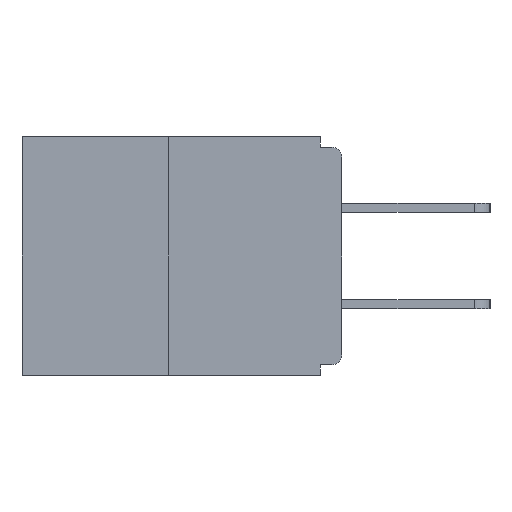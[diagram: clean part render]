
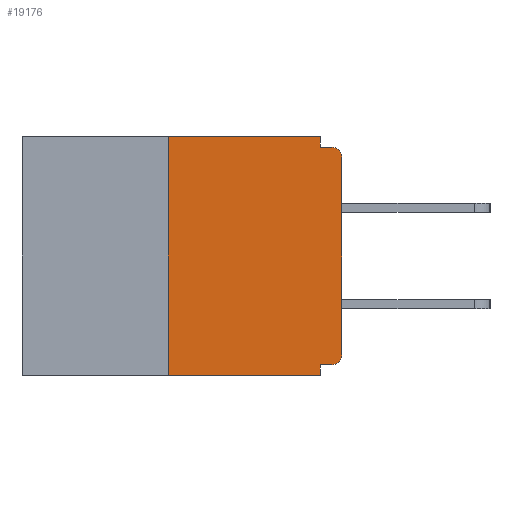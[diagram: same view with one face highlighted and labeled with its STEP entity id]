
A CAD part, left-side view. The second image highlights one B-rep face of the part: STEP entity #19176.
In plain terms, the highlighted planar face has unit normal (-1, 0, 0).
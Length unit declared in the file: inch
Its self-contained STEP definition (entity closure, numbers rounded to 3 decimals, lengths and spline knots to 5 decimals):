
#109 = VECTOR ( 'NONE', #12124, 39.37008 ) ;
#890 = DIRECTION ( 'NONE',  ( 0., 0., -1. ) ) ;
#1224 = VERTEX_POINT ( 'NONE', #20344 ) ;
#1294 = DIRECTION ( 'NONE',  ( 0., -1., 0. ) ) ;
#1757 = ORIENTED_EDGE ( 'NONE', *, *, #17096, .F. ) ;
#1772 = VERTEX_POINT ( 'NONE', #9847 ) ;
#1871 = CARTESIAN_POINT ( 'NONE',  ( 0., 0.46, -0.343 ) ) ;
#2047 = EDGE_CURVE ( 'NONE', #1772, #11818, #23178, .T. ) ;
#2252 = VERTEX_POINT ( 'NONE', #16601 ) ;
#2496 = CARTESIAN_POINT ( 'NONE',  ( 0., 0.015, -0.313 ) ) ;
#2564 = LINE ( 'NONE', #8183, #4224 ) ;
#2820 = EDGE_LOOP ( 'NONE', ( #18465, #4068, #4355, #13558, #8547, #20188, #20332, #4637, #1757, #14184 ) ) ;
#2982 = CARTESIAN_POINT ( 'NONE',  ( 0., 0.015, -0.015 ) ) ;
#3089 = CARTESIAN_POINT ( 'NONE',  ( 0., 0.46, 0. ) ) ;
#3506 = DIRECTION ( 'NONE',  ( 0., 0., -1. ) ) ;
#3647 = DIRECTION ( 'NONE',  ( 0., -1., 0. ) ) ;
#3712 = DIRECTION ( 'NONE',  ( -1., 0., 0. ) ) ;
#4068 = ORIENTED_EDGE ( 'NONE', *, *, #13432, .F. ) ;
#4129 = AXIS2_PLACEMENT_3D ( 'NONE', #2496, #11666, #890 ) ;
#4168 = EDGE_CURVE ( 'NONE', #21518, #18926, #2564, .T. ) ;
#4224 = VECTOR ( 'NONE', #11991, 39.37008 ) ;
#4355 = ORIENTED_EDGE ( 'NONE', *, *, #15649, .T. ) ;
#4608 = VERTEX_POINT ( 'NONE', #17874 ) ;
#4637 = ORIENTED_EDGE ( 'NONE', *, *, #2047, .T. ) ;
#4979 = PLANE ( 'NONE',  #14099 ) ;
#5808 = CARTESIAN_POINT ( 'NONE',  ( 0., 0., 0. ) ) ;
#6082 = DIRECTION ( 'NONE',  ( 0., 0., -1. ) ) ;
#7068 = VERTEX_POINT ( 'NONE', #15095 ) ;
#7612 = LINE ( 'NONE', #1871, #18264 ) ;
#7613 = DIRECTION ( 'NONE',  ( 0., 0., 1. ) ) ;
#8183 = CARTESIAN_POINT ( 'NONE',  ( 0., 0., -0.328 ) ) ;
#8504 = DIRECTION ( 'NONE',  ( 1., 0., 0. ) ) ;
#8547 = ORIENTED_EDGE ( 'NONE', *, *, #4168, .F. ) ;
#9450 = CARTESIAN_POINT ( 'NONE',  ( 0., 0.031, -0.015 ) ) ;
#9847 = CARTESIAN_POINT ( 'NONE',  ( 0., 0., -0.03 ) ) ;
#11199 = CARTESIAN_POINT ( 'NONE',  ( 0., 0.015, -0.328 ) ) ;
#11535 = LINE ( 'NONE', #3089, #15716 ) ;
#11554 = EDGE_CURVE ( 'NONE', #2252, #21466, #13607, .T. ) ;
#11607 = FACE_OUTER_BOUND ( 'NONE', #2820, .T. ) ;
#11666 = DIRECTION ( 'NONE',  ( -1., 0., 0. ) ) ;
#11818 = VERTEX_POINT ( 'NONE', #2982 ) ;
#11991 = DIRECTION ( 'NONE',  ( 0., 1., 0. ) ) ;
#12065 = VECTOR ( 'NONE', #6082, 39.37008 ) ;
#12124 = DIRECTION ( 'NONE',  ( 0., 0., 1. ) ) ;
#12547 = DIRECTION ( 'NONE',  ( 0., -1., 0. ) ) ;
#13024 = CARTESIAN_POINT ( 'NONE',  ( 0., 0.031, -0.328 ) ) ;
#13432 = EDGE_CURVE ( 'NONE', #4608, #13611, #20861, .T. ) ;
#13506 = CARTESIAN_POINT ( 'NONE',  ( 0., 0.25, 0. ) ) ;
#13558 = ORIENTED_EDGE ( 'NONE', *, *, #21403, .F. ) ;
#13607 = LINE ( 'NONE', #16676, #16184 ) ;
#13611 = VERTEX_POINT ( 'NONE', #13506 ) ;
#13874 = CARTESIAN_POINT ( 'NONE',  ( 0., 0.46, 0. ) ) ;
#14099 = AXIS2_PLACEMENT_3D ( 'NONE', #13874, #8504, #3506 ) ;
#14184 = ORIENTED_EDGE ( 'NONE', *, *, #11554, .F. ) ;
#14550 = DIRECTION ( 'NONE',  ( 0., 0., -1. ) ) ;
#14556 = CARTESIAN_POINT ( 'NONE',  ( 0., 0.031, -0.343 ) ) ;
#15095 = CARTESIAN_POINT ( 'NONE',  ( 0., 0., -0.313 ) ) ;
#15246 = EDGE_CURVE ( 'NONE', #21518, #7068, #22780, .T. ) ;
#15649 = EDGE_CURVE ( 'NONE', #4608, #1224, #7612, .T. ) ;
#15716 = VECTOR ( 'NONE', #1294, 39.37008 ) ;
#16184 = VECTOR ( 'NONE', #20270, 39.37008 ) ;
#16260 = VECTOR ( 'NONE', #12547, 39.37008 ) ;
#16422 = EDGE_CURVE ( 'NONE', #13611, #2252, #11535, .T. ) ;
#16601 = CARTESIAN_POINT ( 'NONE',  ( 0., 0.031, 0. ) ) ;
#16676 = CARTESIAN_POINT ( 'NONE',  ( 0., 0.031, 0. ) ) ;
#16879 = LINE ( 'NONE', #5808, #19947 ) ;
#17096 = EDGE_CURVE ( 'NONE', #21466, #11818, #21308, .T. ) ;
#17874 = CARTESIAN_POINT ( 'NONE',  ( 0., 0.25, -0.343 ) ) ;
#18264 = VECTOR ( 'NONE', #3647, 39.37008 ) ;
#18465 = ORIENTED_EDGE ( 'NONE', *, *, #16422, .F. ) ;
#18926 = VERTEX_POINT ( 'NONE', #13024 ) ;
#19035 = LINE ( 'NONE', #14556, #12065 ) ;
#19176 = ADVANCED_FACE ( 'NONE', ( #11607 ), #4979, .F. ) ;
#19384 = CARTESIAN_POINT ( 'NONE',  ( 0., 0.25, 0. ) ) ;
#19947 = VECTOR ( 'NONE', #7613, 39.37008 ) ;
#20188 = ORIENTED_EDGE ( 'NONE', *, *, #15246, .T. ) ;
#20270 = DIRECTION ( 'NONE',  ( 0., 0., -1. ) ) ;
#20332 = ORIENTED_EDGE ( 'NONE', *, *, #20353, .T. ) ;
#20344 = CARTESIAN_POINT ( 'NONE',  ( 0., 0.031, -0.343 ) ) ;
#20353 = EDGE_CURVE ( 'NONE', #7068, #1772, #16879, .T. ) ;
#20861 = LINE ( 'NONE', #19384, #109 ) ;
#21308 = LINE ( 'NONE', #21420, #16260 ) ;
#21403 = EDGE_CURVE ( 'NONE', #18926, #1224, #19035, .T. ) ;
#21420 = CARTESIAN_POINT ( 'NONE',  ( 0., 0., -0.015 ) ) ;
#21465 = CARTESIAN_POINT ( 'NONE',  ( 0., 0.015, -0.03 ) ) ;
#21466 = VERTEX_POINT ( 'NONE', #9450 ) ;
#21518 = VERTEX_POINT ( 'NONE', #11199 ) ;
#21736 = AXIS2_PLACEMENT_3D ( 'NONE', #21465, #3712, #14550 ) ;
#22780 = CIRCLE ( 'NONE', #4129, 0.015 ) ;
#23178 = CIRCLE ( 'NONE', #21736, 0.015 ) ;
